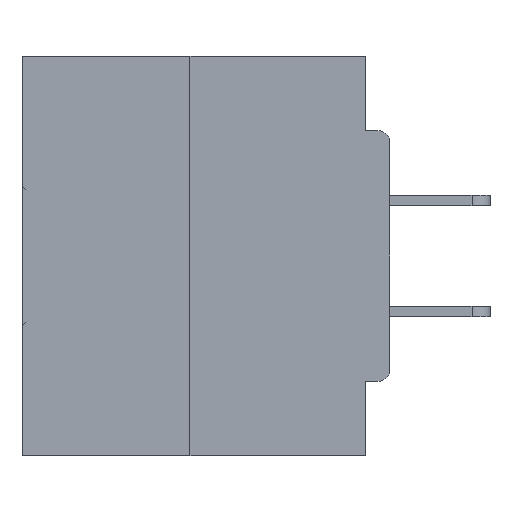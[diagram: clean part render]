
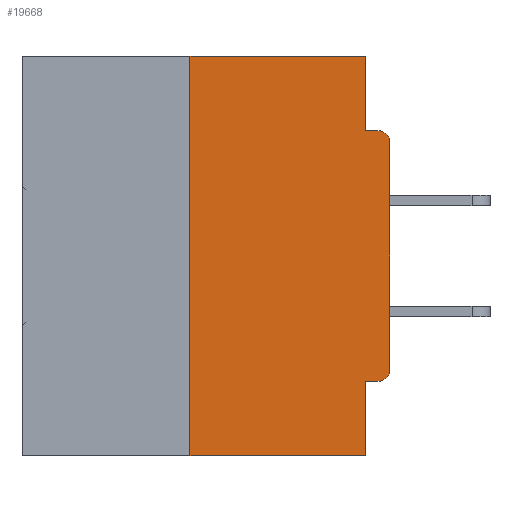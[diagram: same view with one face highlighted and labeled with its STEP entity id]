
A CAD part, left-side view. The second image highlights one B-rep face of the part: STEP entity #19668.
In plain terms, the highlighted planar face has unit normal (-1, 0, 0).
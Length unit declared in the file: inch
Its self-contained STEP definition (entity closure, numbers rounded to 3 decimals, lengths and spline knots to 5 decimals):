
#700 = DIRECTION ( 'NONE',  ( 0., -1., 0. ) ) ;
#2046 = ORIENTED_EDGE ( 'NONE', *, *, #17503, .F. ) ;
#3040 = AXIS2_PLACEMENT_3D ( 'NONE', #32464, #42664, #29006 ) ;
#3346 = LINE ( 'NONE', #18590, #12606 ) ;
#3809 = VECTOR ( 'NONE', #36000, 39.37008 ) ;
#6073 = EDGE_CURVE ( 'NONE', #6310, #17836, #39345, .T. ) ;
#6194 = VECTOR ( 'NONE', #700, 39.37008 ) ;
#6310 = VERTEX_POINT ( 'NONE', #14680 ) ;
#6827 = DIRECTION ( 'NONE',  ( -1., 0., 0. ) ) ;
#6943 = LINE ( 'NONE', #40407, #8519 ) ;
#7506 = VECTOR ( 'NONE', #18249, 39.37008 ) ;
#7578 = VERTEX_POINT ( 'NONE', #42038 ) ;
#7919 = CARTESIAN_POINT ( 'NONE',  ( 0., 0., -0.3915 ) ) ;
#8519 = VECTOR ( 'NONE', #26908, 39.37008 ) ;
#8580 = ORIENTED_EDGE ( 'NONE', *, *, #26454, .F. ) ;
#8801 = ORIENTED_EDGE ( 'NONE', *, *, #6073, .T. ) ;
#9512 = CARTESIAN_POINT ( 'NONE',  ( 0., 0.031, -0.0935 ) ) ;
#9855 = VERTEX_POINT ( 'NONE', #7919 ) ;
#11513 = CARTESIAN_POINT ( 'NONE',  ( 0., 0., 0. ) ) ;
#11659 = EDGE_CURVE ( 'NONE', #9855, #6310, #12673, .T. ) ;
#12547 = EDGE_CURVE ( 'NONE', #40406, #19529, #12600, .T. ) ;
#12572 = CARTESIAN_POINT ( 'NONE',  ( 0., 0.031, -0.5 ) ) ;
#12600 = LINE ( 'NONE', #17233, #3809 ) ;
#12606 = VECTOR ( 'NONE', #18882, 39.37008 ) ;
#12673 = LINE ( 'NONE', #11513, #21484 ) ;
#12869 = AXIS2_PLACEMENT_3D ( 'NONE', #15597, #21862, #13139 ) ;
#13139 = DIRECTION ( 'NONE',  ( 0., 0., -1. ) ) ;
#14224 = ORIENTED_EDGE ( 'NONE', *, *, #25173, .F. ) ;
#14440 = CARTESIAN_POINT ( 'NONE',  ( 0., 0., -0.4065 ) ) ;
#14680 = CARTESIAN_POINT ( 'NONE',  ( 0., 0., -0.1085 ) ) ;
#15272 = VERTEX_POINT ( 'NONE', #23876 ) ;
#15426 = DIRECTION ( 'NONE',  ( 0., -1., 0. ) ) ;
#15597 = CARTESIAN_POINT ( 'NONE',  ( 0., 0.015, -0.1085 ) ) ;
#15716 = EDGE_LOOP ( 'NONE', ( #21780, #28427, #23994, #25567, #8580, #36667, #30707, #8801, #14224, #2046 ) ) ;
#16458 = DIRECTION ( 'NONE',  ( 0., 0., -1. ) ) ;
#16843 = CARTESIAN_POINT ( 'NONE',  ( 0., 0.015, -0.0935 ) ) ;
#17017 = CIRCLE ( 'NONE', #41471, 0.015 ) ;
#17233 = CARTESIAN_POINT ( 'NONE',  ( 0., 0.25, 0. ) ) ;
#17503 = EDGE_CURVE ( 'NONE', #7578, #40481, #6943, .T. ) ;
#17696 = VECTOR ( 'NONE', #15426, 39.37008 ) ;
#17836 = VERTEX_POINT ( 'NONE', #16843 ) ;
#18249 = DIRECTION ( 'NONE',  ( 0., 0., -1. ) ) ;
#18590 = CARTESIAN_POINT ( 'NONE',  ( 0., 0.46, 0. ) ) ;
#18882 = DIRECTION ( 'NONE',  ( 0., -1., 0. ) ) ;
#19529 = VERTEX_POINT ( 'NONE', #36695 ) ;
#19668 = ADVANCED_FACE ( 'NONE', ( #42394 ), #23925, .F. ) ;
#19680 = VERTEX_POINT ( 'NONE', #12572 ) ;
#21484 = VECTOR ( 'NONE', #37741, 39.37008 ) ;
#21780 = ORIENTED_EDGE ( 'NONE', *, *, #33606, .F. ) ;
#21862 = DIRECTION ( 'NONE',  ( -1., 0., 0. ) ) ;
#22268 = VECTOR ( 'NONE', #36954, 39.37008 ) ;
#23723 = LINE ( 'NONE', #36863, #6194 ) ;
#23876 = CARTESIAN_POINT ( 'NONE',  ( 0., 0.031, -0.4065 ) ) ;
#23925 = PLANE ( 'NONE',  #3040 ) ;
#23994 = ORIENTED_EDGE ( 'NONE', *, *, #39567, .T. ) ;
#24183 = VERTEX_POINT ( 'NONE', #30980 ) ;
#25173 = EDGE_CURVE ( 'NONE', #40481, #17836, #40923, .T. ) ;
#25567 = ORIENTED_EDGE ( 'NONE', *, *, #41890, .F. ) ;
#26454 = EDGE_CURVE ( 'NONE', #24183, #15272, #39744, .T. ) ;
#26908 = DIRECTION ( 'NONE',  ( 0., 0., -1. ) ) ;
#27666 = LINE ( 'NONE', #39160, #7506 ) ;
#28427 = ORIENTED_EDGE ( 'NONE', *, *, #12547, .F. ) ;
#29006 = DIRECTION ( 'NONE',  ( 0., 0., -1. ) ) ;
#30707 = ORIENTED_EDGE ( 'NONE', *, *, #11659, .T. ) ;
#30980 = CARTESIAN_POINT ( 'NONE',  ( 0., 0.015, -0.4065 ) ) ;
#32464 = CARTESIAN_POINT ( 'NONE',  ( 0., 0.46, 0. ) ) ;
#32991 = EDGE_CURVE ( 'NONE', #24183, #9855, #17017, .T. ) ;
#33606 = EDGE_CURVE ( 'NONE', #19529, #7578, #3346, .T. ) ;
#35049 = CARTESIAN_POINT ( 'NONE',  ( 0., 0.25, -0.5 ) ) ;
#36000 = DIRECTION ( 'NONE',  ( 0., 0., 1. ) ) ;
#36667 = ORIENTED_EDGE ( 'NONE', *, *, #32991, .T. ) ;
#36695 = CARTESIAN_POINT ( 'NONE',  ( 0., 0.25, 0. ) ) ;
#36863 = CARTESIAN_POINT ( 'NONE',  ( 0., 0.46, -0.5 ) ) ;
#36954 = DIRECTION ( 'NONE',  ( 0., 1., 0. ) ) ;
#37741 = DIRECTION ( 'NONE',  ( 0., 0., 1. ) ) ;
#39079 = CARTESIAN_POINT ( 'NONE',  ( 0., 0., -0.0935 ) ) ;
#39160 = CARTESIAN_POINT ( 'NONE',  ( 0., 0.031, -0.5 ) ) ;
#39345 = CIRCLE ( 'NONE', #12869, 0.015 ) ;
#39567 = EDGE_CURVE ( 'NONE', #40406, #19680, #23723, .T. ) ;
#39744 = LINE ( 'NONE', #14440, #22268 ) ;
#40101 = CARTESIAN_POINT ( 'NONE',  ( 0., 0.015, -0.3915 ) ) ;
#40406 = VERTEX_POINT ( 'NONE', #35049 ) ;
#40407 = CARTESIAN_POINT ( 'NONE',  ( 0., 0.031, 0. ) ) ;
#40481 = VERTEX_POINT ( 'NONE', #9512 ) ;
#40923 = LINE ( 'NONE', #39079, #17696 ) ;
#41471 = AXIS2_PLACEMENT_3D ( 'NONE', #40101, #6827, #16458 ) ;
#41890 = EDGE_CURVE ( 'NONE', #15272, #19680, #27666, .T. ) ;
#42038 = CARTESIAN_POINT ( 'NONE',  ( 0., 0.031, 0. ) ) ;
#42394 = FACE_OUTER_BOUND ( 'NONE', #15716, .T. ) ;
#42664 = DIRECTION ( 'NONE',  ( 1., 0., 0. ) ) ;
